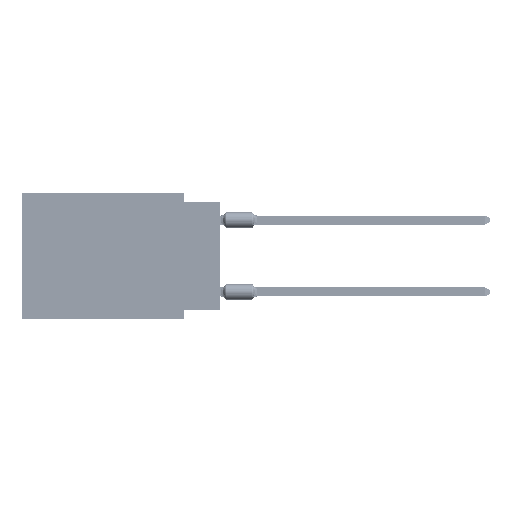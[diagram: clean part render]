
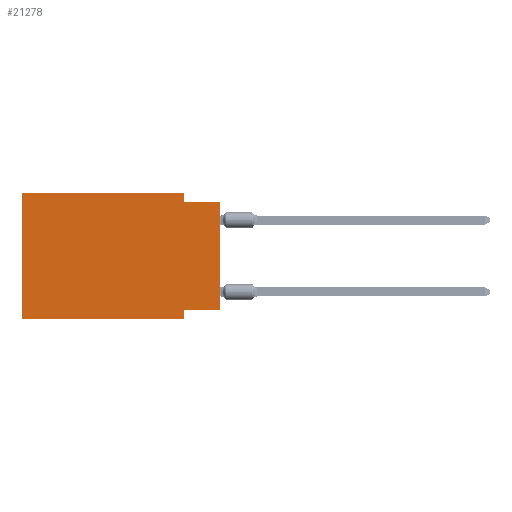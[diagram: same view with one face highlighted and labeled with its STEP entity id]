
A CAD part, left-side view. The second image highlights one B-rep face of the part: STEP entity #21278.
In plain terms, the highlighted planar face has unit normal (-1, 0, 0).
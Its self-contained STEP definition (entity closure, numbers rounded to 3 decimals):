
#1351 = CARTESIAN_POINT ( 'NONE',  ( 0., 0., -8.255 ) ) ;
#1848 = LINE ( 'NONE', #1351, #18648 ) ;
#4601 = LINE ( 'NONE', #92242, #84443 ) ;
#5031 = CARTESIAN_POINT ( 'NONE',  ( 0., 0., -0.635 ) ) ;
#5418 = VECTOR ( 'NONE', #11341, 1000. ) ;
#5767 = CARTESIAN_POINT ( 'NONE',  ( 0., 13.97, 0. ) ) ;
#6758 = CARTESIAN_POINT ( 'NONE',  ( 0., 0., -8.255 ) ) ;
#9141 = CARTESIAN_POINT ( 'NONE',  ( 0., 0., -0.635 ) ) ;
#9383 = EDGE_CURVE ( 'NONE', #63999, #29538, #71601, .T. ) ;
#11341 = DIRECTION ( 'NONE',  ( 0., -1., 0. ) ) ;
#11843 = LINE ( 'NONE', #44748, #5418 ) ;
#12987 = VERTEX_POINT ( 'NONE', #5031 ) ;
#13592 = PLANE ( 'NONE',  #38187 ) ;
#14106 = EDGE_CURVE ( 'NONE', #34243, #63999, #11843, .T. ) ;
#15665 = VERTEX_POINT ( 'NONE', #86482 ) ;
#18259 = DIRECTION ( 'NONE',  ( 0., 0., 1. ) ) ;
#18648 = VECTOR ( 'NONE', #97330, 1000. ) ;
#19694 = VECTOR ( 'NONE', #25855, 1000. ) ;
#19763 = DIRECTION ( 'NONE',  ( 0., 0., 1. ) ) ;
#20183 = ORIENTED_EDGE ( 'NONE', *, *, #14106, .F. ) ;
#20220 = EDGE_CURVE ( 'NONE', #69679, #34243, #4601, .T. ) ;
#20414 = DIRECTION ( 'NONE',  ( 1., 0., 0. ) ) ;
#21278 = ADVANCED_FACE ( 'NONE', ( #85063 ), #13592, .F. ) ;
#21565 = ORIENTED_EDGE ( 'NONE', *, *, #96249, .F. ) ;
#24565 = LINE ( 'NONE', #56369, #102660 ) ;
#25305 = ORIENTED_EDGE ( 'NONE', *, *, #96169, .F. ) ;
#25855 = DIRECTION ( 'NONE',  ( 0., -1., 0. ) ) ;
#28351 = ORIENTED_EDGE ( 'NONE', *, *, #94046, .T. ) ;
#28659 = LINE ( 'NONE', #89731, #84917 ) ;
#29538 = VERTEX_POINT ( 'NONE', #89876 ) ;
#34243 = VERTEX_POINT ( 'NONE', #87745 ) ;
#34579 = VERTEX_POINT ( 'NONE', #6758 ) ;
#38187 = AXIS2_PLACEMENT_3D ( 'NONE', #5767, #20414, #85574 ) ;
#39196 = DIRECTION ( 'NONE',  ( 0., -1., 0. ) ) ;
#42840 = VERTEX_POINT ( 'NONE', #67598 ) ;
#44240 = ORIENTED_EDGE ( 'NONE', *, *, #66038, .F. ) ;
#44748 = CARTESIAN_POINT ( 'NONE',  ( 0., 13.97, 0. ) ) ;
#48154 = CARTESIAN_POINT ( 'NONE',  ( 0., 13.97, -8.89 ) ) ;
#50084 = ORIENTED_EDGE ( 'NONE', *, *, #20220, .F. ) ;
#56369 = CARTESIAN_POINT ( 'NONE',  ( 0., 13.97, -8.89 ) ) ;
#56635 = DIRECTION ( 'NONE',  ( 0., 0., -1. ) ) ;
#58162 = LINE ( 'NONE', #9141, #19694 ) ;
#61934 = ORIENTED_EDGE ( 'NONE', *, *, #82728, .T. ) ;
#63999 = VERTEX_POINT ( 'NONE', #67438 ) ;
#66038 = EDGE_CURVE ( 'NONE', #34579, #15665, #1848, .T. ) ;
#67438 = CARTESIAN_POINT ( 'NONE',  ( 0., 2.54, 0. ) ) ;
#67598 = CARTESIAN_POINT ( 'NONE',  ( 0., 2.54, -8.89 ) ) ;
#69020 = EDGE_LOOP ( 'NONE', ( #61934, #21565, #100321, #20183, #50084, #28351, #25305, #44240 ) ) ;
#69679 = VERTEX_POINT ( 'NONE', #48154 ) ;
#70577 = CARTESIAN_POINT ( 'NONE',  ( 0., 2.54, 0. ) ) ;
#71248 = CARTESIAN_POINT ( 'NONE',  ( 0., 2.54, -8.89 ) ) ;
#71601 = LINE ( 'NONE', #70577, #87713 ) ;
#72108 = DIRECTION ( 'NONE',  ( 0., 0., -1. ) ) ;
#79087 = LINE ( 'NONE', #71248, #79626 ) ;
#79626 = VECTOR ( 'NONE', #56635, 1000. ) ;
#82728 = EDGE_CURVE ( 'NONE', #34579, #12987, #28659, .T. ) ;
#84443 = VECTOR ( 'NONE', #19763, 1000. ) ;
#84917 = VECTOR ( 'NONE', #18259, 1000. ) ;
#85063 = FACE_OUTER_BOUND ( 'NONE', #69020, .T. ) ;
#85574 = DIRECTION ( 'NONE',  ( 0., 0., -1. ) ) ;
#86482 = CARTESIAN_POINT ( 'NONE',  ( 0., 2.54, -8.255 ) ) ;
#87713 = VECTOR ( 'NONE', #72108, 1000. ) ;
#87745 = CARTESIAN_POINT ( 'NONE',  ( 0., 13.97, 0. ) ) ;
#89731 = CARTESIAN_POINT ( 'NONE',  ( 0., 0., 0. ) ) ;
#89876 = CARTESIAN_POINT ( 'NONE',  ( 0., 2.54, -0.635 ) ) ;
#92242 = CARTESIAN_POINT ( 'NONE',  ( 0., 13.97, 0. ) ) ;
#94046 = EDGE_CURVE ( 'NONE', #69679, #42840, #24565, .T. ) ;
#96169 = EDGE_CURVE ( 'NONE', #15665, #42840, #79087, .T. ) ;
#96249 = EDGE_CURVE ( 'NONE', #29538, #12987, #58162, .T. ) ;
#97330 = DIRECTION ( 'NONE',  ( 0., 1., 0. ) ) ;
#100321 = ORIENTED_EDGE ( 'NONE', *, *, #9383, .F. ) ;
#102660 = VECTOR ( 'NONE', #39196, 1000. ) ;
